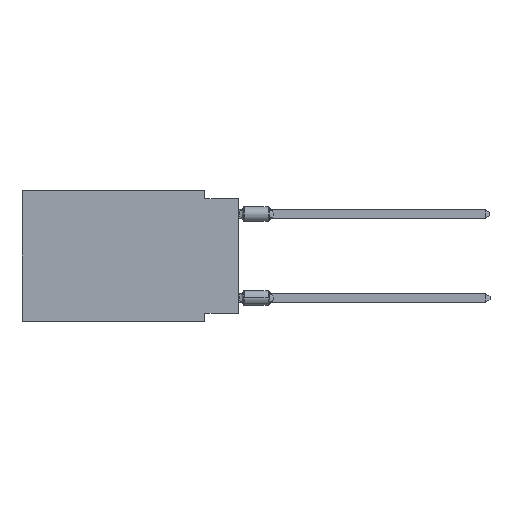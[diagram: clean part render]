
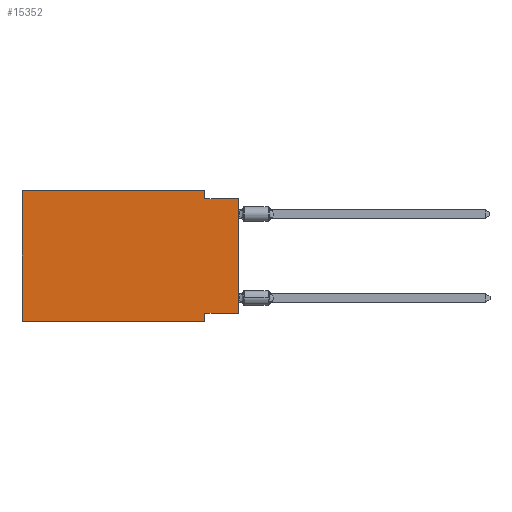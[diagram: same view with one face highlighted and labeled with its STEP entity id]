
A CAD part, left-side view. The second image highlights one B-rep face of the part: STEP entity #15352.
In plain terms, the highlighted planar face has unit normal (-1, 0, 0).
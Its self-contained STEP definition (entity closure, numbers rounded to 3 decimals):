
#162 = LINE ( 'NONE', #17948, #17592 ) ;
#661 = VECTOR ( 'NONE', #28104, 1000. ) ;
#741 = EDGE_CURVE ( 'NONE', #26443, #2708, #17980, .T. ) ;
#1222 = VECTOR ( 'NONE', #15914, 1000. ) ;
#1325 = CARTESIAN_POINT ( 'NONE',  ( 0., 0., -9.271 ) ) ;
#1902 = VECTOR ( 'NONE', #17657, 1000. ) ;
#2142 = VERTEX_POINT ( 'NONE', #1325 ) ;
#2189 = VERTEX_POINT ( 'NONE', #21092 ) ;
#2708 = VERTEX_POINT ( 'NONE', #9973 ) ;
#2813 = CARTESIAN_POINT ( 'NONE',  ( 0., 16.383, 0. ) ) ;
#3033 = EDGE_CURVE ( 'NONE', #28756, #14559, #8294, .T. ) ;
#3716 = ORIENTED_EDGE ( 'NONE', *, *, #5041, .F. ) ;
#4923 = EDGE_CURVE ( 'NONE', #2142, #2189, #162, .T. ) ;
#5041 = EDGE_CURVE ( 'NONE', #9353, #14559, #12347, .T. ) ;
#5191 = DIRECTION ( 'NONE',  ( 0., 0., -1. ) ) ;
#5200 = CARTESIAN_POINT ( 'NONE',  ( 0., 0., -0.635 ) ) ;
#5411 = ORIENTED_EDGE ( 'NONE', *, *, #7830, .F. ) ;
#5934 = DIRECTION ( 'NONE',  ( 0., 1., 0. ) ) ;
#6006 = EDGE_LOOP ( 'NONE', ( #28636, #5411, #7719, #27103, #18869, #6795, #3716, #16296 ) ) ;
#6024 = CARTESIAN_POINT ( 'NONE',  ( 0., 2.54, 0. ) ) ;
#6795 = ORIENTED_EDGE ( 'NONE', *, *, #3033, .T. ) ;
#7575 = DIRECTION ( 'NONE',  ( 0., 0., 1. ) ) ;
#7719 = ORIENTED_EDGE ( 'NONE', *, *, #10234, .F. ) ;
#7830 = EDGE_CURVE ( 'NONE', #32525, #2189, #30755, .T. ) ;
#7965 = LINE ( 'NONE', #22974, #661 ) ;
#8294 = LINE ( 'NONE', #8447, #16435 ) ;
#8447 = CARTESIAN_POINT ( 'NONE',  ( 0., 16.383, -9.906 ) ) ;
#8735 = LINE ( 'NONE', #24060, #22770 ) ;
#9353 = VERTEX_POINT ( 'NONE', #27931 ) ;
#9383 = EDGE_CURVE ( 'NONE', #28756, #26443, #7965, .T. ) ;
#9877 = DIRECTION ( 'NONE',  ( 0., 0., -1. ) ) ;
#9973 = CARTESIAN_POINT ( 'NONE',  ( 0., 2.54, 0. ) ) ;
#9993 = EDGE_CURVE ( 'NONE', #2142, #9353, #8735, .T. ) ;
#10129 = AXIS2_PLACEMENT_3D ( 'NONE', #19523, #17382, #5191 ) ;
#10234 = EDGE_CURVE ( 'NONE', #2708, #32525, #18377, .T. ) ;
#11248 = DIRECTION ( 'NONE',  ( 0., -1., 0. ) ) ;
#12347 = LINE ( 'NONE', #22399, #31825 ) ;
#14559 = VERTEX_POINT ( 'NONE', #20266 ) ;
#15352 = ADVANCED_FACE ( 'NONE', ( #27794 ), #25149, .F. ) ;
#15914 = DIRECTION ( 'NONE',  ( 0., 0., -1. ) ) ;
#16296 = ORIENTED_EDGE ( 'NONE', *, *, #9993, .F. ) ;
#16435 = VECTOR ( 'NONE', #11248, 1000. ) ;
#17382 = DIRECTION ( 'NONE',  ( 1., 0., 0. ) ) ;
#17592 = VECTOR ( 'NONE', #7575, 1000. ) ;
#17657 = DIRECTION ( 'NONE',  ( 0., -1., 0. ) ) ;
#17948 = CARTESIAN_POINT ( 'NONE',  ( 0., 0., 0. ) ) ;
#17980 = LINE ( 'NONE', #2813, #1902 ) ;
#18377 = LINE ( 'NONE', #6024, #1222 ) ;
#18869 = ORIENTED_EDGE ( 'NONE', *, *, #9383, .F. ) ;
#19523 = CARTESIAN_POINT ( 'NONE',  ( 0., 16.383, 0. ) ) ;
#19580 = VECTOR ( 'NONE', #30581, 1000. ) ;
#20266 = CARTESIAN_POINT ( 'NONE',  ( 0., 2.54, -9.906 ) ) ;
#21092 = CARTESIAN_POINT ( 'NONE',  ( 0., 0., -0.635 ) ) ;
#22339 = CARTESIAN_POINT ( 'NONE',  ( 0., 16.383, -9.906 ) ) ;
#22399 = CARTESIAN_POINT ( 'NONE',  ( 0., 2.54, -9.906 ) ) ;
#22770 = VECTOR ( 'NONE', #5934, 1000. ) ;
#22974 = CARTESIAN_POINT ( 'NONE',  ( 0., 16.383, 0. ) ) ;
#23436 = CARTESIAN_POINT ( 'NONE',  ( 0., 16.383, 0. ) ) ;
#24060 = CARTESIAN_POINT ( 'NONE',  ( 0., 0., -9.271 ) ) ;
#24274 = CARTESIAN_POINT ( 'NONE',  ( 0., 2.54, -0.635 ) ) ;
#25149 = PLANE ( 'NONE',  #10129 ) ;
#26443 = VERTEX_POINT ( 'NONE', #23436 ) ;
#27103 = ORIENTED_EDGE ( 'NONE', *, *, #741, .F. ) ;
#27794 = FACE_OUTER_BOUND ( 'NONE', #6006, .T. ) ;
#27931 = CARTESIAN_POINT ( 'NONE',  ( 0., 2.54, -9.271 ) ) ;
#28104 = DIRECTION ( 'NONE',  ( 0., 0., 1. ) ) ;
#28636 = ORIENTED_EDGE ( 'NONE', *, *, #4923, .T. ) ;
#28756 = VERTEX_POINT ( 'NONE', #22339 ) ;
#30581 = DIRECTION ( 'NONE',  ( 0., -1., 0. ) ) ;
#30755 = LINE ( 'NONE', #5200, #19580 ) ;
#31825 = VECTOR ( 'NONE', #9877, 1000. ) ;
#32525 = VERTEX_POINT ( 'NONE', #24274 ) ;
